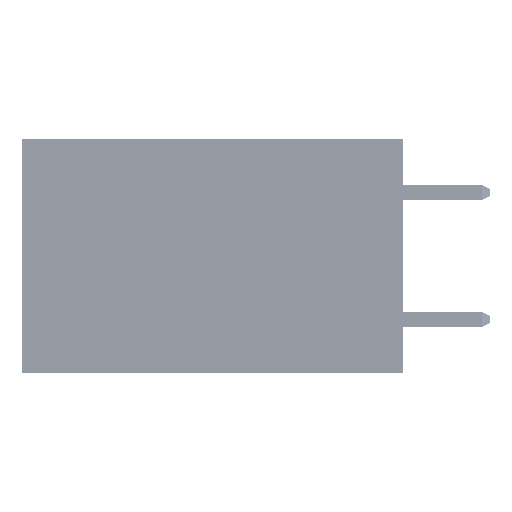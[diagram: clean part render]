
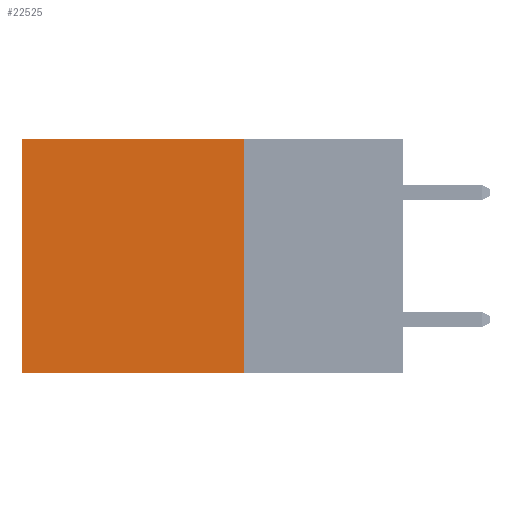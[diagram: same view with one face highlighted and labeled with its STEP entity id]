
A CAD part, left-side view. The second image highlights one B-rep face of the part: STEP entity #22525.
In plain terms, the highlighted planar face has unit normal (-1, 0, 0).
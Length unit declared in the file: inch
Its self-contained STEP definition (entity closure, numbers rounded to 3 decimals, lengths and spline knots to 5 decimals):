
#1428 = CARTESIAN_POINT ( 'NONE',  ( 0.2875, 0.6, -0.37 ) ) ;
#5614 = EDGE_LOOP ( 'NONE', ( #41177, #34507, #29557, #16492 ) ) ;
#5918 = CARTESIAN_POINT ( 'NONE',  ( 0.2875, 0.25, 0. ) ) ;
#8067 = EDGE_CURVE ( 'NONE', #36086, #46135, #9422, .T. ) ;
#8830 = EDGE_CURVE ( 'NONE', #31041, #36827, #46717, .T. ) ;
#9135 = AXIS2_PLACEMENT_3D ( 'NONE', #30580, #14992, #19131 ) ;
#9247 = CARTESIAN_POINT ( 'NONE',  ( 0.2875, 0.6, 0. ) ) ;
#9422 = LINE ( 'NONE', #9247, #21828 ) ;
#11130 = VECTOR ( 'NONE', #32885, 39.37008 ) ;
#14992 = DIRECTION ( 'NONE',  ( 1., 0., 0. ) ) ;
#16492 = ORIENTED_EDGE ( 'NONE', *, *, #20738, .T. ) ;
#18787 = VECTOR ( 'NONE', #46896, 39.37008 ) ;
#19049 = CARTESIAN_POINT ( 'NONE',  ( 0.2875, 0.25, -0.37 ) ) ;
#19131 = DIRECTION ( 'NONE',  ( 0., 0., -1. ) ) ;
#20738 = EDGE_CURVE ( 'NONE', #31041, #36086, #34227, .T. ) ;
#21828 = VECTOR ( 'NONE', #28413, 39.37008 ) ;
#22525 = ADVANCED_FACE ( 'NONE', ( #46533 ), #45875, .F. ) ;
#22684 = DIRECTION ( 'NONE',  ( 0., 1., 0. ) ) ;
#25169 = CARTESIAN_POINT ( 'NONE',  ( 0.2875, 0.25, 0. ) ) ;
#28413 = DIRECTION ( 'NONE',  ( 0., 0., -1. ) ) ;
#29557 = ORIENTED_EDGE ( 'NONE', *, *, #8830, .F. ) ;
#30580 = CARTESIAN_POINT ( 'NONE',  ( 0.2875, 0.25, 0. ) ) ;
#31041 = VERTEX_POINT ( 'NONE', #45368 ) ;
#31722 = EDGE_CURVE ( 'NONE', #36827, #46135, #41837, .T. ) ;
#32885 = DIRECTION ( 'NONE',  ( 0., 0., -1. ) ) ;
#34227 = LINE ( 'NONE', #5918, #18787 ) ;
#34507 = ORIENTED_EDGE ( 'NONE', *, *, #31722, .F. ) ;
#36086 = VERTEX_POINT ( 'NONE', #36746 ) ;
#36746 = CARTESIAN_POINT ( 'NONE',  ( 0.2875, 0.6, 0. ) ) ;
#36827 = VERTEX_POINT ( 'NONE', #41649 ) ;
#38894 = VECTOR ( 'NONE', #22684, 39.37008 ) ;
#41177 = ORIENTED_EDGE ( 'NONE', *, *, #8067, .T. ) ;
#41649 = CARTESIAN_POINT ( 'NONE',  ( 0.2875, 0.25, -0.37 ) ) ;
#41837 = LINE ( 'NONE', #19049, #38894 ) ;
#45368 = CARTESIAN_POINT ( 'NONE',  ( 0.2875, 0.25, 0. ) ) ;
#45875 = PLANE ( 'NONE',  #9135 ) ;
#46135 = VERTEX_POINT ( 'NONE', #1428 ) ;
#46533 = FACE_OUTER_BOUND ( 'NONE', #5614, .T. ) ;
#46717 = LINE ( 'NONE', #25169, #11130 ) ;
#46896 = DIRECTION ( 'NONE',  ( 0., 1., 0. ) ) ;
